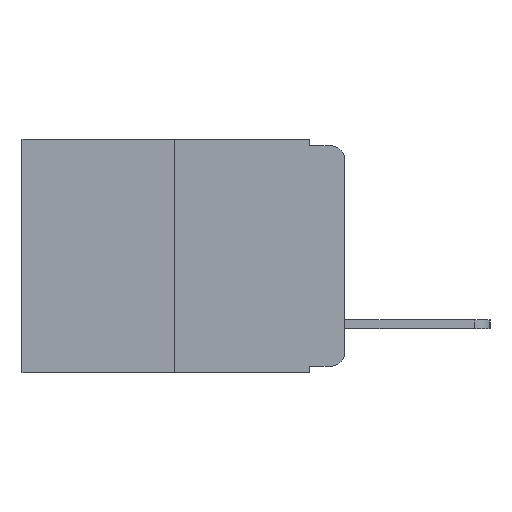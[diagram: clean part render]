
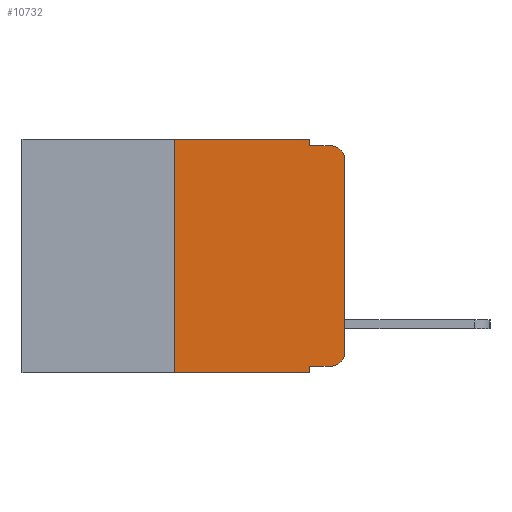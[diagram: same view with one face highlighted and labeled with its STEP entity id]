
A CAD part, left-side view. The second image highlights one B-rep face of the part: STEP entity #10732.
In plain terms, the highlighted planar face has unit normal (-1, 0, 0).
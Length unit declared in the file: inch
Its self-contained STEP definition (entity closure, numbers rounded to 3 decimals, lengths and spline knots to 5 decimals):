
#68 = CARTESIAN_POINT ( 'NONE',  ( 0., 0.02, -0.333 ) ) ;
#141 = LINE ( 'NONE', #7312, #2548 ) ;
#289 = VERTEX_POINT ( 'NONE', #9223 ) ;
#331 = DIRECTION ( 'NONE',  ( 0., 0., -1. ) ) ;
#492 = EDGE_CURVE ( 'NONE', #8947, #8656, #8852, .T. ) ;
#578 = VECTOR ( 'NONE', #6366, 39.37008 ) ;
#589 = LINE ( 'NONE', #4422, #5830 ) ;
#920 = DIRECTION ( 'NONE',  ( 0., 0., 1. ) ) ;
#969 = ORIENTED_EDGE ( 'NONE', *, *, #9563, .F. ) ;
#1016 = DIRECTION ( 'NONE',  ( 0., 0., 1. ) ) ;
#1158 = VERTEX_POINT ( 'NONE', #11984 ) ;
#1423 = VECTOR ( 'NONE', #920, 39.37008 ) ;
#1703 = CIRCLE ( 'NONE', #8432, 0.02 ) ;
#1947 = ORIENTED_EDGE ( 'NONE', *, *, #10222, .T. ) ;
#1953 = DIRECTION ( 'NONE',  ( 0., -1., 0. ) ) ;
#2268 = CARTESIAN_POINT ( 'NONE',  ( 0., 0.051, 0. ) ) ;
#2548 = VECTOR ( 'NONE', #8244, 39.37008 ) ;
#2778 = LINE ( 'NONE', #11487, #7869 ) ;
#2834 = VERTEX_POINT ( 'NONE', #7675 ) ;
#3032 = CARTESIAN_POINT ( 'NONE',  ( 0., 0., -0.313 ) ) ;
#3293 = LINE ( 'NONE', #10068, #578 ) ;
#3763 = DIRECTION ( 'NONE',  ( -1., 0., 0. ) ) ;
#3766 = EDGE_CURVE ( 'NONE', #2834, #8638, #1703, .T. ) ;
#3964 = ORIENTED_EDGE ( 'NONE', *, *, #10642, .T. ) ;
#4109 = VECTOR ( 'NONE', #5680, 39.37008 ) ;
#4422 = CARTESIAN_POINT ( 'NONE',  ( 0., 0.473, -0.343 ) ) ;
#4550 = DIRECTION ( 'NONE',  ( 1., 0., 0. ) ) ;
#4658 = FACE_OUTER_BOUND ( 'NONE', #7955, .T. ) ;
#4967 = CARTESIAN_POINT ( 'NONE',  ( 0., 0.051, -0.01 ) ) ;
#5438 = EDGE_CURVE ( 'NONE', #6119, #8638, #2778, .T. ) ;
#5680 = DIRECTION ( 'NONE',  ( 0., -1., 0. ) ) ;
#5823 = CARTESIAN_POINT ( 'NONE',  ( 0., 0., 0. ) ) ;
#5830 = VECTOR ( 'NONE', #10083, 39.37008 ) ;
#5890 = ORIENTED_EDGE ( 'NONE', *, *, #5438, .F. ) ;
#6119 = VERTEX_POINT ( 'NONE', #4967 ) ;
#6244 = DIRECTION ( 'NONE',  ( -1., 0., 0. ) ) ;
#6249 = VERTEX_POINT ( 'NONE', #6994 ) ;
#6313 = CARTESIAN_POINT ( 'NONE',  ( 0., 0.051, -0.333 ) ) ;
#6366 = DIRECTION ( 'NONE',  ( 0., 0., -1. ) ) ;
#6777 = ORIENTED_EDGE ( 'NONE', *, *, #492, .T. ) ;
#6994 = CARTESIAN_POINT ( 'NONE',  ( 0., 0.051, 0. ) ) ;
#7312 = CARTESIAN_POINT ( 'NONE',  ( 0., 0.473, 0. ) ) ;
#7367 = PLANE ( 'NONE',  #11549 ) ;
#7675 = CARTESIAN_POINT ( 'NONE',  ( 0., 0., -0.03 ) ) ;
#7831 = CARTESIAN_POINT ( 'NONE',  ( 0., 0.25, 0. ) ) ;
#7832 = ORIENTED_EDGE ( 'NONE', *, *, #10336, .T. ) ;
#7869 = VECTOR ( 'NONE', #1953, 39.37008 ) ;
#7870 = CARTESIAN_POINT ( 'NONE',  ( 0., 0.02, -0.01 ) ) ;
#7944 = VERTEX_POINT ( 'NONE', #3032 ) ;
#7955 = EDGE_LOOP ( 'NONE', ( #7832, #10611, #5890, #8409, #969, #8711, #3964, #11481, #6777, #1947 ) ) ;
#7980 = VECTOR ( 'NONE', #8965, 39.37008 ) ;
#8244 = DIRECTION ( 'NONE',  ( 0., -1., 0. ) ) ;
#8374 = VERTEX_POINT ( 'NONE', #12138 ) ;
#8409 = ORIENTED_EDGE ( 'NONE', *, *, #8728, .F. ) ;
#8432 = AXIS2_PLACEMENT_3D ( 'NONE', #11864, #6244, #331 ) ;
#8612 = EDGE_CURVE ( 'NONE', #289, #1158, #11345, .T. ) ;
#8638 = VERTEX_POINT ( 'NONE', #7870 ) ;
#8656 = VERTEX_POINT ( 'NONE', #68 ) ;
#8711 = ORIENTED_EDGE ( 'NONE', *, *, #8612, .F. ) ;
#8728 = EDGE_CURVE ( 'NONE', #6249, #6119, #9880, .T. ) ;
#8852 = LINE ( 'NONE', #6313, #4109 ) ;
#8947 = VERTEX_POINT ( 'NONE', #12080 ) ;
#8965 = DIRECTION ( 'NONE',  ( 0., 0., -1. ) ) ;
#9223 = CARTESIAN_POINT ( 'NONE',  ( 0., 0.25, -0.343 ) ) ;
#9428 = CARTESIAN_POINT ( 'NONE',  ( 0., 0.02, -0.313 ) ) ;
#9510 = AXIS2_PLACEMENT_3D ( 'NONE', #9428, #3763, #10372 ) ;
#9563 = EDGE_CURVE ( 'NONE', #1158, #6249, #141, .T. ) ;
#9880 = LINE ( 'NONE', #2268, #7980 ) ;
#10068 = CARTESIAN_POINT ( 'NONE',  ( 0., 0.051, 0. ) ) ;
#10083 = DIRECTION ( 'NONE',  ( 0., -1., 0. ) ) ;
#10202 = CARTESIAN_POINT ( 'NONE',  ( 0., 0.473, 0. ) ) ;
#10222 = EDGE_CURVE ( 'NONE', #8656, #7944, #10572, .T. ) ;
#10336 = EDGE_CURVE ( 'NONE', #7944, #2834, #11587, .T. ) ;
#10372 = DIRECTION ( 'NONE',  ( 0., 0., -1. ) ) ;
#10572 = CIRCLE ( 'NONE', #9510, 0.02 ) ;
#10611 = ORIENTED_EDGE ( 'NONE', *, *, #3766, .T. ) ;
#10642 = EDGE_CURVE ( 'NONE', #289, #8374, #589, .T. ) ;
#10732 = ADVANCED_FACE ( 'NONE', ( #4658 ), #7367, .F. ) ;
#11135 = DIRECTION ( 'NONE',  ( 0., 0., -1. ) ) ;
#11345 = LINE ( 'NONE', #7831, #11632 ) ;
#11481 = ORIENTED_EDGE ( 'NONE', *, *, #11745, .F. ) ;
#11487 = CARTESIAN_POINT ( 'NONE',  ( 0., 0.051, -0.01 ) ) ;
#11549 = AXIS2_PLACEMENT_3D ( 'NONE', #10202, #4550, #11135 ) ;
#11587 = LINE ( 'NONE', #5823, #1423 ) ;
#11632 = VECTOR ( 'NONE', #1016, 39.37008 ) ;
#11745 = EDGE_CURVE ( 'NONE', #8947, #8374, #3293, .T. ) ;
#11864 = CARTESIAN_POINT ( 'NONE',  ( 0., 0.02, -0.03 ) ) ;
#11984 = CARTESIAN_POINT ( 'NONE',  ( 0., 0.25, 0. ) ) ;
#12080 = CARTESIAN_POINT ( 'NONE',  ( 0., 0.051, -0.333 ) ) ;
#12138 = CARTESIAN_POINT ( 'NONE',  ( 0., 0.051, -0.343 ) ) ;
